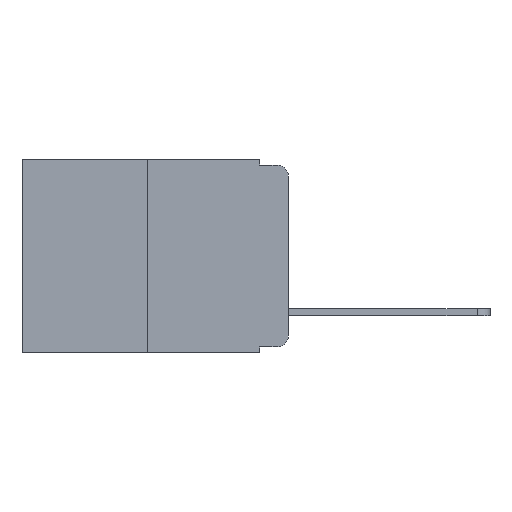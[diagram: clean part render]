
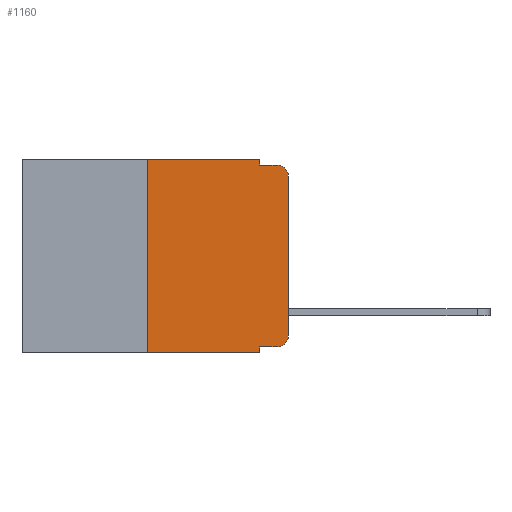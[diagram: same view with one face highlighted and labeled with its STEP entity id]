
A CAD part, left-side view. The second image highlights one B-rep face of the part: STEP entity #1160.
In plain terms, the highlighted planar face has unit normal (-1, 0, 0).
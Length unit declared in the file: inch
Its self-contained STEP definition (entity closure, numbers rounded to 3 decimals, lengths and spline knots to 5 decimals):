
#182 = ORIENTED_EDGE ( 'NONE', *, *, #5360, .T. ) ;
#392 = EDGE_CURVE ( 'NONE', #6873, #2931, #8434, .T. ) ;
#594 = EDGE_LOOP ( 'NONE', ( #4702, #8647, #7465, #4726, #730, #8892, #1159, #4579, #1003, #182 ) ) ;
#679 = LINE ( 'NONE', #686, #9746 ) ;
#686 = CARTESIAN_POINT ( 'NONE',  ( 0., 0.051, -0.333 ) ) ;
#730 = ORIENTED_EDGE ( 'NONE', *, *, #11298, .F. ) ;
#746 = LINE ( 'NONE', #3893, #9810 ) ;
#998 = VERTEX_POINT ( 'NONE', #2084 ) ;
#1003 = ORIENTED_EDGE ( 'NONE', *, *, #9954, .T. ) ;
#1073 = VECTOR ( 'NONE', #4798, 39.37008 ) ;
#1159 = ORIENTED_EDGE ( 'NONE', *, *, #4464, .T. ) ;
#1160 = ADVANCED_FACE ( 'NONE', ( #2499 ), #6412, .F. ) ;
#1220 = DIRECTION ( 'NONE',  ( 0., -1., 0. ) ) ;
#1353 = VECTOR ( 'NONE', #7167, 39.37008 ) ;
#1605 = DIRECTION ( 'NONE',  ( -1., 0., 0. ) ) ;
#1641 = LINE ( 'NONE', #2728, #1353 ) ;
#1717 = VECTOR ( 'NONE', #5373, 39.37008 ) ;
#2014 = LINE ( 'NONE', #5913, #1717 ) ;
#2084 = CARTESIAN_POINT ( 'NONE',  ( 0., 0., -0.03 ) ) ;
#2499 = FACE_OUTER_BOUND ( 'NONE', #594, .T. ) ;
#2540 = AXIS2_PLACEMENT_3D ( 'NONE', #8273, #7731, #6659 ) ;
#2586 = CARTESIAN_POINT ( 'NONE',  ( 0., 0.25, -0.343 ) ) ;
#2728 = CARTESIAN_POINT ( 'NONE',  ( 0., 0.473, 0. ) ) ;
#2931 = VERTEX_POINT ( 'NONE', #6786 ) ;
#3015 = CARTESIAN_POINT ( 'NONE',  ( 0., 0.051, 0. ) ) ;
#3215 = VERTEX_POINT ( 'NONE', #6889 ) ;
#3258 = VERTEX_POINT ( 'NONE', #3916 ) ;
#3335 = EDGE_CURVE ( 'NONE', #5684, #998, #2014, .T. ) ;
#3480 = DIRECTION ( 'NONE',  ( -1., 0., 0. ) ) ;
#3893 = CARTESIAN_POINT ( 'NONE',  ( 0., 0.051, -0.01 ) ) ;
#3916 = CARTESIAN_POINT ( 'NONE',  ( 0., 0.02, -0.01 ) ) ;
#3941 = LINE ( 'NONE', #9981, #8335 ) ;
#3977 = DIRECTION ( 'NONE',  ( 0., -1., 0. ) ) ;
#4092 = EDGE_CURVE ( 'NONE', #6574, #7249, #3941, .T. ) ;
#4314 = DIRECTION ( 'NONE',  ( 0., -1., 0. ) ) ;
#4464 = EDGE_CURVE ( 'NONE', #6574, #2931, #4822, .T. ) ;
#4514 = VECTOR ( 'NONE', #3977, 39.37008 ) ;
#4579 = ORIENTED_EDGE ( 'NONE', *, *, #392, .F. ) ;
#4702 = ORIENTED_EDGE ( 'NONE', *, *, #3335, .T. ) ;
#4726 = ORIENTED_EDGE ( 'NONE', *, *, #10878, .F. ) ;
#4796 = CARTESIAN_POINT ( 'NONE',  ( 0., 0.051, -0.333 ) ) ;
#4798 = DIRECTION ( 'NONE',  ( 0., 0., -1. ) ) ;
#4822 = LINE ( 'NONE', #5789, #4514 ) ;
#5360 = EDGE_CURVE ( 'NONE', #7642, #5684, #7270, .T. ) ;
#5373 = DIRECTION ( 'NONE',  ( 0., 0., 1. ) ) ;
#5684 = VERTEX_POINT ( 'NONE', #5807 ) ;
#5789 = CARTESIAN_POINT ( 'NONE',  ( 0., 0.473, -0.343 ) ) ;
#5807 = CARTESIAN_POINT ( 'NONE',  ( 0., 0., -0.313 ) ) ;
#5913 = CARTESIAN_POINT ( 'NONE',  ( 0., 0., 0. ) ) ;
#5929 = EDGE_CURVE ( 'NONE', #998, #3258, #8182, .T. ) ;
#6044 = VERTEX_POINT ( 'NONE', #6320 ) ;
#6154 = VECTOR ( 'NONE', #9125, 39.37008 ) ;
#6320 = CARTESIAN_POINT ( 'NONE',  ( 0., 0.051, -0.01 ) ) ;
#6412 = PLANE ( 'NONE',  #2540 ) ;
#6436 = CARTESIAN_POINT ( 'NONE',  ( 0., 0.051, 0. ) ) ;
#6574 = VERTEX_POINT ( 'NONE', #2586 ) ;
#6659 = DIRECTION ( 'NONE',  ( 0., 0., -1. ) ) ;
#6786 = CARTESIAN_POINT ( 'NONE',  ( 0., 0.051, -0.343 ) ) ;
#6873 = VERTEX_POINT ( 'NONE', #4796 ) ;
#6889 = CARTESIAN_POINT ( 'NONE',  ( 0., 0.051, 0. ) ) ;
#6990 = CARTESIAN_POINT ( 'NONE',  ( 0., 0.02, -0.313 ) ) ;
#7016 = DIRECTION ( 'NONE',  ( 0., 0., 1. ) ) ;
#7167 = DIRECTION ( 'NONE',  ( 0., -1., 0. ) ) ;
#7249 = VERTEX_POINT ( 'NONE', #7415 ) ;
#7270 = CIRCLE ( 'NONE', #9983, 0.02 ) ;
#7415 = CARTESIAN_POINT ( 'NONE',  ( 0., 0.25, 0. ) ) ;
#7465 = ORIENTED_EDGE ( 'NONE', *, *, #8511, .F. ) ;
#7642 = VERTEX_POINT ( 'NONE', #9651 ) ;
#7731 = DIRECTION ( 'NONE',  ( 1., 0., 0. ) ) ;
#7834 = DIRECTION ( 'NONE',  ( 0., 0., -1. ) ) ;
#8182 = CIRCLE ( 'NONE', #9022, 0.02 ) ;
#8273 = CARTESIAN_POINT ( 'NONE',  ( 0., 0.473, 0. ) ) ;
#8335 = VECTOR ( 'NONE', #7016, 39.37008 ) ;
#8434 = LINE ( 'NONE', #6436, #1073 ) ;
#8511 = EDGE_CURVE ( 'NONE', #6044, #3258, #746, .T. ) ;
#8647 = ORIENTED_EDGE ( 'NONE', *, *, #5929, .T. ) ;
#8741 = CARTESIAN_POINT ( 'NONE',  ( 0., 0.02, -0.03 ) ) ;
#8892 = ORIENTED_EDGE ( 'NONE', *, *, #4092, .F. ) ;
#9022 = AXIS2_PLACEMENT_3D ( 'NONE', #8741, #3480, #9567 ) ;
#9125 = DIRECTION ( 'NONE',  ( 0., 0., -1. ) ) ;
#9567 = DIRECTION ( 'NONE',  ( 0., 0., -1. ) ) ;
#9651 = CARTESIAN_POINT ( 'NONE',  ( 0., 0.02, -0.333 ) ) ;
#9746 = VECTOR ( 'NONE', #4314, 39.37008 ) ;
#9810 = VECTOR ( 'NONE', #1220, 39.37008 ) ;
#9954 = EDGE_CURVE ( 'NONE', #6873, #7642, #679, .T. ) ;
#9981 = CARTESIAN_POINT ( 'NONE',  ( 0., 0.25, 0. ) ) ;
#9983 = AXIS2_PLACEMENT_3D ( 'NONE', #6990, #1605, #7834 ) ;
#10623 = LINE ( 'NONE', #3015, #6154 ) ;
#10878 = EDGE_CURVE ( 'NONE', #3215, #6044, #10623, .T. ) ;
#11298 = EDGE_CURVE ( 'NONE', #7249, #3215, #1641, .T. ) ;
